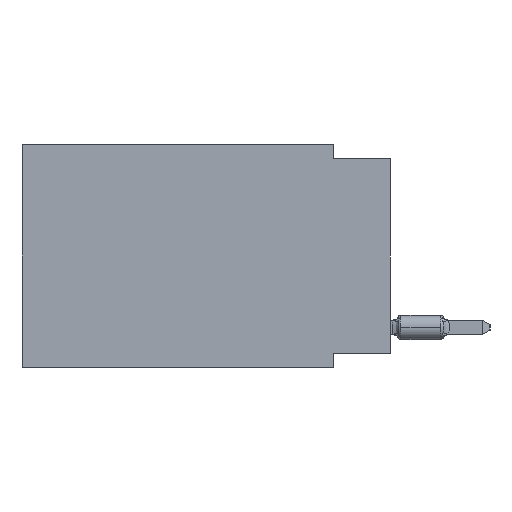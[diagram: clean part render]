
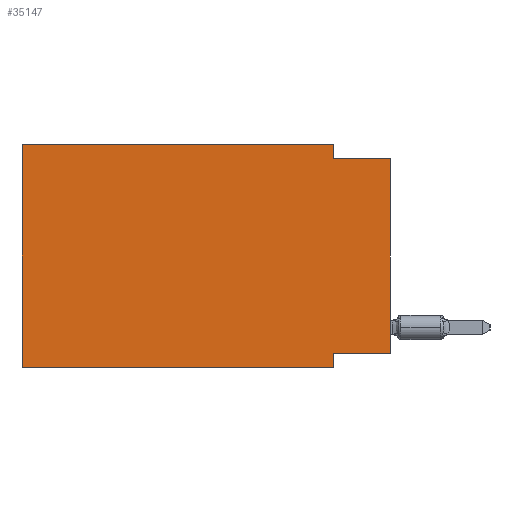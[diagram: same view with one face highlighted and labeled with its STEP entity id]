
A CAD part, left-side view. The second image highlights one B-rep face of the part: STEP entity #35147.
In plain terms, the highlighted planar face has unit normal (-1, 0, 0).
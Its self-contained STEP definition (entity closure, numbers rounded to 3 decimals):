
#429 = CARTESIAN_POINT ( 'NONE',  ( 0., 2.54, -9.906 ) ) ;
#1344 = VERTEX_POINT ( 'NONE', #17725 ) ;
#1994 = ORIENTED_EDGE ( 'NONE', *, *, #41345, .F. ) ;
#2044 = ORIENTED_EDGE ( 'NONE', *, *, #31488, .T. ) ;
#3132 = LINE ( 'NONE', #26924, #14561 ) ;
#3356 = VECTOR ( 'NONE', #6674, 1000. ) ;
#3927 = CARTESIAN_POINT ( 'NONE',  ( 0., 16.383, -9.906 ) ) ;
#4823 = ORIENTED_EDGE ( 'NONE', *, *, #35395, .F. ) ;
#6067 = VERTEX_POINT ( 'NONE', #29897 ) ;
#6219 = VERTEX_POINT ( 'NONE', #48092 ) ;
#6674 = DIRECTION ( 'NONE',  ( 0., 0., -1. ) ) ;
#8178 = ORIENTED_EDGE ( 'NONE', *, *, #45761, .F. ) ;
#11333 = DIRECTION ( 'NONE',  ( 0., -1., 0. ) ) ;
#12403 = LINE ( 'NONE', #3927, #48379 ) ;
#13210 = VERTEX_POINT ( 'NONE', #25087 ) ;
#13757 = EDGE_CURVE ( 'NONE', #13210, #6067, #13778, .T. ) ;
#13778 = LINE ( 'NONE', #14049, #14557 ) ;
#14049 = CARTESIAN_POINT ( 'NONE',  ( 0., 0., -9.271 ) ) ;
#14557 = VECTOR ( 'NONE', #30713, 1000. ) ;
#14561 = VECTOR ( 'NONE', #11333, 1000. ) ;
#17086 = DIRECTION ( 'NONE',  ( 0., 0., -1. ) ) ;
#17531 = ORIENTED_EDGE ( 'NONE', *, *, #13757, .F. ) ;
#17725 = CARTESIAN_POINT ( 'NONE',  ( 0., 2.54, 0. ) ) ;
#18991 = CARTESIAN_POINT ( 'NONE',  ( 0., 2.54, 0. ) ) ;
#20609 = DIRECTION ( 'NONE',  ( 0., -1., 0. ) ) ;
#20714 = EDGE_CURVE ( 'NONE', #6067, #24526, #37793, .T. ) ;
#22293 = VERTEX_POINT ( 'NONE', #50333 ) ;
#22627 = FACE_OUTER_BOUND ( 'NONE', #28861, .T. ) ;
#23601 = CARTESIAN_POINT ( 'NONE',  ( 0., 0., -0.635 ) ) ;
#24526 = VERTEX_POINT ( 'NONE', #38522 ) ;
#25087 = CARTESIAN_POINT ( 'NONE',  ( 0., 0., -9.271 ) ) ;
#26924 = CARTESIAN_POINT ( 'NONE',  ( 0., 16.383, 0. ) ) ;
#27020 = VECTOR ( 'NONE', #17086, 1000. ) ;
#27914 = LINE ( 'NONE', #35833, #30500 ) ;
#28255 = VERTEX_POINT ( 'NONE', #48873 ) ;
#28861 = EDGE_LOOP ( 'NONE', ( #2044, #8178, #50105, #1994, #4823, #32432, #47095, #17531 ) ) ;
#29713 = VERTEX_POINT ( 'NONE', #45564 ) ;
#29751 = EDGE_CURVE ( 'NONE', #1344, #22293, #39687, .T. ) ;
#29897 = CARTESIAN_POINT ( 'NONE',  ( 0., 2.54, -9.271 ) ) ;
#30260 = PLANE ( 'NONE',  #48913 ) ;
#30500 = VECTOR ( 'NONE', #40433, 1000. ) ;
#30713 = DIRECTION ( 'NONE',  ( 0., 1., 0. ) ) ;
#31488 = EDGE_CURVE ( 'NONE', #13210, #6219, #27914, .T. ) ;
#32432 = ORIENTED_EDGE ( 'NONE', *, *, #52098, .T. ) ;
#35147 = ADVANCED_FACE ( 'NONE', ( #22627 ), #30260, .F. ) ;
#35395 = EDGE_CURVE ( 'NONE', #29713, #28255, #41115, .T. ) ;
#35833 = CARTESIAN_POINT ( 'NONE',  ( 0., 0., 0. ) ) ;
#36366 = VECTOR ( 'NONE', #52962, 1000. ) ;
#37624 = VECTOR ( 'NONE', #41381, 1000. ) ;
#37793 = LINE ( 'NONE', #429, #27020 ) ;
#38522 = CARTESIAN_POINT ( 'NONE',  ( 0., 2.54, -9.906 ) ) ;
#38980 = DIRECTION ( 'NONE',  ( 1., 0., 0. ) ) ;
#39687 = LINE ( 'NONE', #18991, #3356 ) ;
#40433 = DIRECTION ( 'NONE',  ( 0., 0., 1. ) ) ;
#41115 = LINE ( 'NONE', #50054, #37624 ) ;
#41345 = EDGE_CURVE ( 'NONE', #28255, #1344, #3132, .T. ) ;
#41381 = DIRECTION ( 'NONE',  ( 0., 0., 1. ) ) ;
#43059 = CARTESIAN_POINT ( 'NONE',  ( 0., 16.383, 0. ) ) ;
#44277 = LINE ( 'NONE', #23601, #36366 ) ;
#45564 = CARTESIAN_POINT ( 'NONE',  ( 0., 16.383, -9.906 ) ) ;
#45761 = EDGE_CURVE ( 'NONE', #22293, #6219, #44277, .T. ) ;
#46845 = DIRECTION ( 'NONE',  ( 0., 0., -1. ) ) ;
#47095 = ORIENTED_EDGE ( 'NONE', *, *, #20714, .F. ) ;
#48092 = CARTESIAN_POINT ( 'NONE',  ( 0., 0., -0.635 ) ) ;
#48379 = VECTOR ( 'NONE', #20609, 1000. ) ;
#48873 = CARTESIAN_POINT ( 'NONE',  ( 0., 16.383, 0. ) ) ;
#48913 = AXIS2_PLACEMENT_3D ( 'NONE', #43059, #38980, #46845 ) ;
#50054 = CARTESIAN_POINT ( 'NONE',  ( 0., 16.383, 0. ) ) ;
#50105 = ORIENTED_EDGE ( 'NONE', *, *, #29751, .F. ) ;
#50333 = CARTESIAN_POINT ( 'NONE',  ( 0., 2.54, -0.635 ) ) ;
#52098 = EDGE_CURVE ( 'NONE', #29713, #24526, #12403, .T. ) ;
#52962 = DIRECTION ( 'NONE',  ( 0., -1., 0. ) ) ;
